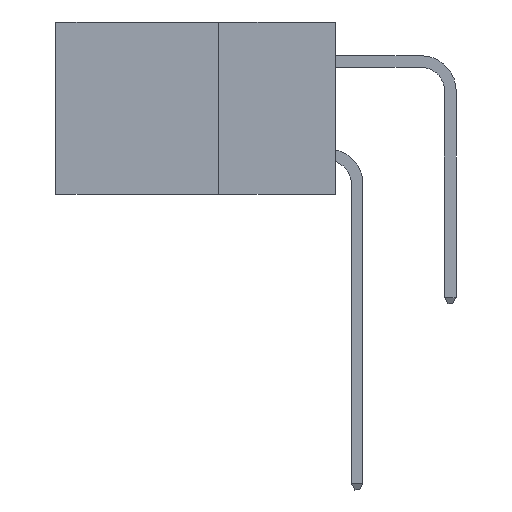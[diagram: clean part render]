
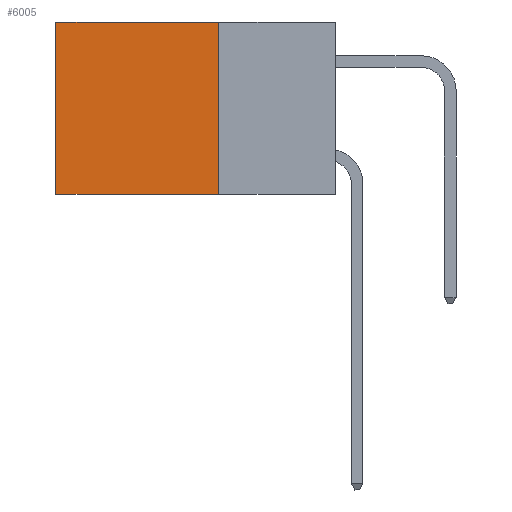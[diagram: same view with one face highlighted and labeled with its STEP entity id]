
A CAD part, left-side view. The second image highlights one B-rep face of the part: STEP entity #6005.
In plain terms, the highlighted planar face has unit normal (-1, 0, 0).
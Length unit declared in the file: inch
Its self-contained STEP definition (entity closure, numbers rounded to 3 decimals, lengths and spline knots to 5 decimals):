
#361 = PLANE ( 'NONE',  #19631 ) ;
#1339 = CARTESIAN_POINT ( 'NONE',  ( 0.2875, 0.25, 0. ) ) ;
#1463 = EDGE_CURVE ( 'NONE', #20193, #17793, #10084, .T. ) ;
#1548 = EDGE_CURVE ( 'NONE', #20272, #17793, #8325, .T. ) ;
#2334 = DIRECTION ( 'NONE',  ( 1., 0., 0. ) ) ;
#3146 = EDGE_LOOP ( 'NONE', ( #12084, #14791, #22737, #13324 ) ) ;
#3172 = CARTESIAN_POINT ( 'NONE',  ( 0.2875, 0.25, 0. ) ) ;
#4055 = FACE_OUTER_BOUND ( 'NONE', #3146, .T. ) ;
#5852 = LINE ( 'NONE', #3172, #10269 ) ;
#6005 = ADVANCED_FACE ( 'NONE', ( #4055 ), #361, .F. ) ;
#6238 = DIRECTION ( 'NONE',  ( 0., 1., 0. ) ) ;
#6264 = VECTOR ( 'NONE', #6238, 39.37008 ) ;
#6407 = CARTESIAN_POINT ( 'NONE',  ( 0.2875, 0.6, 0. ) ) ;
#7680 = VECTOR ( 'NONE', #16869, 39.37008 ) ;
#8325 = LINE ( 'NONE', #6407, #12730 ) ;
#8874 = DIRECTION ( 'NONE',  ( 0., 1., 0. ) ) ;
#10084 = LINE ( 'NONE', #19157, #6264 ) ;
#10269 = VECTOR ( 'NONE', #8874, 39.37008 ) ;
#12084 = ORIENTED_EDGE ( 'NONE', *, *, #1548, .T. ) ;
#12702 = LINE ( 'NONE', #20481, #7680 ) ;
#12730 = VECTOR ( 'NONE', #17479, 39.37008 ) ;
#13324 = ORIENTED_EDGE ( 'NONE', *, *, #16468, .T. ) ;
#13609 = CARTESIAN_POINT ( 'NONE',  ( 0.2875, 0.25, -0.37 ) ) ;
#13624 = CARTESIAN_POINT ( 'NONE',  ( 0.2875, 0.25, 0. ) ) ;
#14791 = ORIENTED_EDGE ( 'NONE', *, *, #1463, .F. ) ;
#15071 = EDGE_CURVE ( 'NONE', #19284, #20193, #12702, .T. ) ;
#15434 = DIRECTION ( 'NONE',  ( 0., 0., -1. ) ) ;
#16468 = EDGE_CURVE ( 'NONE', #19284, #20272, #5852, .T. ) ;
#16869 = DIRECTION ( 'NONE',  ( 0., 0., -1. ) ) ;
#17479 = DIRECTION ( 'NONE',  ( 0., 0., -1. ) ) ;
#17793 = VERTEX_POINT ( 'NONE', #20004 ) ;
#19157 = CARTESIAN_POINT ( 'NONE',  ( 0.2875, 0.25, -0.37 ) ) ;
#19284 = VERTEX_POINT ( 'NONE', #1339 ) ;
#19631 = AXIS2_PLACEMENT_3D ( 'NONE', #13624, #2334, #15434 ) ;
#20004 = CARTESIAN_POINT ( 'NONE',  ( 0.2875, 0.6, -0.37 ) ) ;
#20193 = VERTEX_POINT ( 'NONE', #13609 ) ;
#20272 = VERTEX_POINT ( 'NONE', #21123 ) ;
#20481 = CARTESIAN_POINT ( 'NONE',  ( 0.2875, 0.25, 0. ) ) ;
#21123 = CARTESIAN_POINT ( 'NONE',  ( 0.2875, 0.6, 0. ) ) ;
#22737 = ORIENTED_EDGE ( 'NONE', *, *, #15071, .F. ) ;
